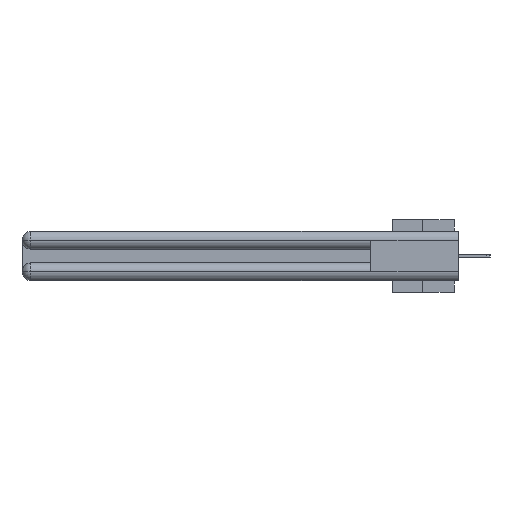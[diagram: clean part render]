
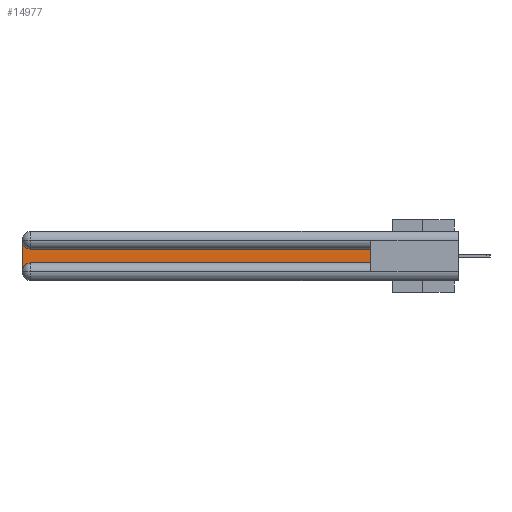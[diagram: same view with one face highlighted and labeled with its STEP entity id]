
A CAD part, left-side view. The second image highlights one B-rep face of the part: STEP entity #14977.
In plain terms, the highlighted planar face has unit normal (-1, 0, 0).
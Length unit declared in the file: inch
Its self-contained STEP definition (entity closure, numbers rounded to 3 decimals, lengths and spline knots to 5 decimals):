
#414 = DIRECTION ( 'NONE',  ( 0., 0., 1. ) ) ;
#828 = VERTEX_POINT ( 'NONE', #9533 ) ;
#987 = CARTESIAN_POINT ( 'NONE',  ( 0.075, 0.6, -0.2175 ) ) ;
#1300 = CARTESIAN_POINT ( 'NONE',  ( 0.075, 3., -0.0625 ) ) ;
#1690 = VECTOR ( 'NONE', #18677, 39.37008 ) ;
#1711 = CARTESIAN_POINT ( 'NONE',  ( 0.075, 3., -0.2175 ) ) ;
#2770 = ORIENTED_EDGE ( 'NONE', *, *, #9357, .T. ) ;
#5167 = CARTESIAN_POINT ( 'NONE',  ( 0.075, 0.6, -0.1225 ) ) ;
#7249 = EDGE_CURVE ( 'NONE', #24578, #13545, #30570, .T. ) ;
#7548 = ORIENTED_EDGE ( 'NONE', *, *, #32865, .T. ) ;
#8114 = AXIS2_PLACEMENT_3D ( 'NONE', #24958, #8243, #27713 ) ;
#8243 = DIRECTION ( 'NONE',  ( 1., 0., 0. ) ) ;
#8578 = VERTEX_POINT ( 'NONE', #27055 ) ;
#9357 = EDGE_CURVE ( 'NONE', #17142, #8578, #18289, .T. ) ;
#9533 = CARTESIAN_POINT ( 'NONE',  ( 0.075, 3., -0.2775 ) ) ;
#11736 = ORIENTED_EDGE ( 'NONE', *, *, #30816, .T. ) ;
#12075 = PLANE ( 'NONE',  #19352 ) ;
#13545 = VERTEX_POINT ( 'NONE', #987 ) ;
#14887 = DIRECTION ( 'NONE',  ( 0., 0., -1. ) ) ;
#14977 = ADVANCED_FACE ( 'NONE', ( #24992 ), #12075, .F. ) ;
#15245 = ORIENTED_EDGE ( 'NONE', *, *, #17127, .T. ) ;
#16352 = VERTEX_POINT ( 'NONE', #1300 ) ;
#16383 = DIRECTION ( 'NONE',  ( 1., 0., 0. ) ) ;
#16601 = CIRCLE ( 'NONE', #35217, 0.06 ) ;
#17022 = CARTESIAN_POINT ( 'NONE',  ( 0.075, 2.94, -0.2175 ) ) ;
#17127 = EDGE_CURVE ( 'NONE', #828, #24578, #25698, .T. ) ;
#17142 = VERTEX_POINT ( 'NONE', #36020 ) ;
#17684 = ORIENTED_EDGE ( 'NONE', *, *, #30710, .T. ) ;
#18193 = LINE ( 'NONE', #33835, #24716 ) ;
#18289 = LINE ( 'NONE', #5167, #32121 ) ;
#18660 = ORIENTED_EDGE ( 'NONE', *, *, #7249, .T. ) ;
#18677 = DIRECTION ( 'NONE',  ( 0., -1., 0. ) ) ;
#18743 = DIRECTION ( 'NONE',  ( 0., 0., -1. ) ) ;
#19352 = AXIS2_PLACEMENT_3D ( 'NONE', #20258, #31460, #14887 ) ;
#19625 = EDGE_LOOP ( 'NONE', ( #2770, #11736, #17684, #15245, #18660, #7548 ) ) ;
#20258 = CARTESIAN_POINT ( 'NONE',  ( 0.075, 3., -0.1225 ) ) ;
#24578 = VERTEX_POINT ( 'NONE', #17022 ) ;
#24716 = VECTOR ( 'NONE', #414, 39.37008 ) ;
#24958 = CARTESIAN_POINT ( 'NONE',  ( 0.075, 2.94, -0.2775 ) ) ;
#24992 = FACE_OUTER_BOUND ( 'NONE', #19625, .T. ) ;
#25698 = CIRCLE ( 'NONE', #8114, 0.06 ) ;
#26632 = VECTOR ( 'NONE', #18743, 39.37008 ) ;
#27055 = CARTESIAN_POINT ( 'NONE',  ( 0.075, 2.94, -0.1225 ) ) ;
#27713 = DIRECTION ( 'NONE',  ( 0., 0., -1. ) ) ;
#29771 = CARTESIAN_POINT ( 'NONE',  ( 0.075, 0.6, -0.2175 ) ) ;
#30289 = DIRECTION ( 'NONE',  ( 0., 1., 0. ) ) ;
#30570 = LINE ( 'NONE', #29771, #1690 ) ;
#30710 = EDGE_CURVE ( 'NONE', #16352, #828, #34786, .T. ) ;
#30816 = EDGE_CURVE ( 'NONE', #8578, #16352, #16601, .T. ) ;
#31460 = DIRECTION ( 'NONE',  ( 1., 0., 0. ) ) ;
#32121 = VECTOR ( 'NONE', #30289, 39.37008 ) ;
#32865 = EDGE_CURVE ( 'NONE', #13545, #17142, #18193, .T. ) ;
#32967 = CARTESIAN_POINT ( 'NONE',  ( 0.075, 2.94, -0.0625 ) ) ;
#33835 = CARTESIAN_POINT ( 'NONE',  ( 0.075, 0.6, -0.2175 ) ) ;
#34786 = LINE ( 'NONE', #1711, #26632 ) ;
#35217 = AXIS2_PLACEMENT_3D ( 'NONE', #32967, #16383, #35741 ) ;
#35741 = DIRECTION ( 'NONE',  ( 0., 0., -1. ) ) ;
#36020 = CARTESIAN_POINT ( 'NONE',  ( 0.075, 0.6, -0.1225 ) ) ;
